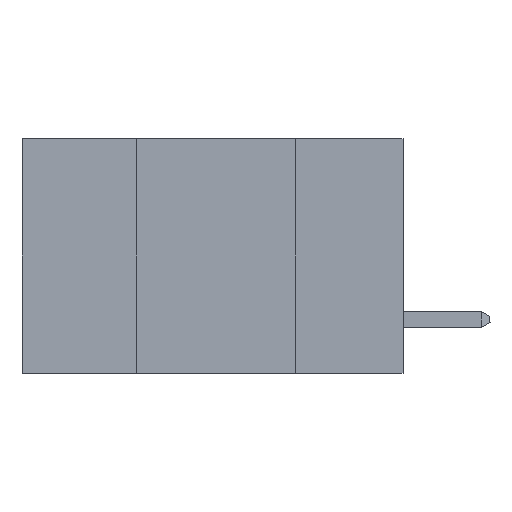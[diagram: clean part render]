
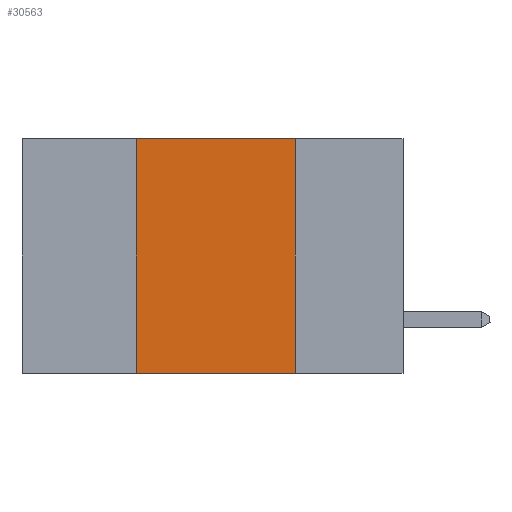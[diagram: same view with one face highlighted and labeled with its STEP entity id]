
A CAD part, left-side view. The second image highlights one B-rep face of the part: STEP entity #30563.
In plain terms, the highlighted planar face has unit normal (-1, 0, 0).
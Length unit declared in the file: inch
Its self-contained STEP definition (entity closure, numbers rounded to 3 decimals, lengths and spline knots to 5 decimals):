
#1395 = VECTOR ( 'NONE', #26885, 39.37008 ) ;
#1993 = CARTESIAN_POINT ( 'NONE',  ( 0., 0.42, 0. ) ) ;
#2172 = DIRECTION ( 'NONE',  ( 0., 0., -1. ) ) ;
#3076 = AXIS2_PLACEMENT_3D ( 'NONE', #11503, #3947, #38369 ) ;
#3240 = LINE ( 'NONE', #4121, #1395 ) ;
#3601 = ORIENTED_EDGE ( 'NONE', *, *, #11056, .F. ) ;
#3810 = VERTEX_POINT ( 'NONE', #1993 ) ;
#3947 = DIRECTION ( 'NONE',  ( 1., 0., 0. ) ) ;
#4121 = CARTESIAN_POINT ( 'NONE',  ( 0., 0.6, -0.37 ) ) ;
#4618 = VECTOR ( 'NONE', #43102, 39.37008 ) ;
#5205 = CARTESIAN_POINT ( 'NONE',  ( 0., 0.17, -0.37 ) ) ;
#7222 = EDGE_CURVE ( 'NONE', #45953, #3810, #44522, .T. ) ;
#7780 = VERTEX_POINT ( 'NONE', #11043 ) ;
#8506 = CARTESIAN_POINT ( 'NONE',  ( 0., 0.6, 0. ) ) ;
#11043 = CARTESIAN_POINT ( 'NONE',  ( 0., 0.17, 0. ) ) ;
#11056 = EDGE_CURVE ( 'NONE', #3810, #7780, #19654, .T. ) ;
#11503 = CARTESIAN_POINT ( 'NONE',  ( 0., 0.6, 0. ) ) ;
#11669 = PLANE ( 'NONE',  #3076 ) ;
#15159 = DIRECTION ( 'NONE',  ( 0., 0., 1. ) ) ;
#19654 = LINE ( 'NONE', #8506, #4618 ) ;
#21832 = ORIENTED_EDGE ( 'NONE', *, *, #34798, .T. ) ;
#23349 = EDGE_CURVE ( 'NONE', #7780, #41924, #38514, .T. ) ;
#26885 = DIRECTION ( 'NONE',  ( 0., -1., 0. ) ) ;
#30563 = ADVANCED_FACE ( 'NONE', ( #49210 ), #11669, .F. ) ;
#33124 = CARTESIAN_POINT ( 'NONE',  ( 0., 0.17, 0. ) ) ;
#34798 = EDGE_CURVE ( 'NONE', #45953, #41924, #3240, .T. ) ;
#37003 = ORIENTED_EDGE ( 'NONE', *, *, #23349, .F. ) ;
#37954 = CARTESIAN_POINT ( 'NONE',  ( 0., 0.42, 0. ) ) ;
#38369 = DIRECTION ( 'NONE',  ( 0., 0., -1. ) ) ;
#38514 = LINE ( 'NONE', #33124, #40314 ) ;
#39767 = VECTOR ( 'NONE', #15159, 39.37008 ) ;
#40314 = VECTOR ( 'NONE', #2172, 39.37008 ) ;
#40867 = EDGE_LOOP ( 'NONE', ( #37003, #3601, #44918, #21832 ) ) ;
#41924 = VERTEX_POINT ( 'NONE', #5205 ) ;
#43102 = DIRECTION ( 'NONE',  ( 0., -1., 0. ) ) ;
#44522 = LINE ( 'NONE', #37954, #39767 ) ;
#44918 = ORIENTED_EDGE ( 'NONE', *, *, #7222, .F. ) ;
#45953 = VERTEX_POINT ( 'NONE', #46240 ) ;
#46240 = CARTESIAN_POINT ( 'NONE',  ( 0., 0.42, -0.37 ) ) ;
#49210 = FACE_OUTER_BOUND ( 'NONE', #40867, .T. ) ;
